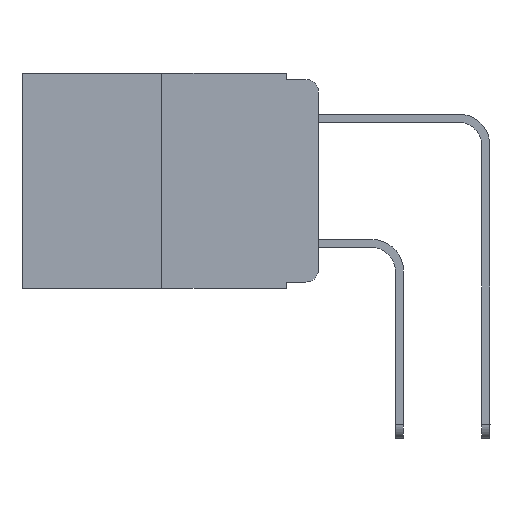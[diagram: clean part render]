
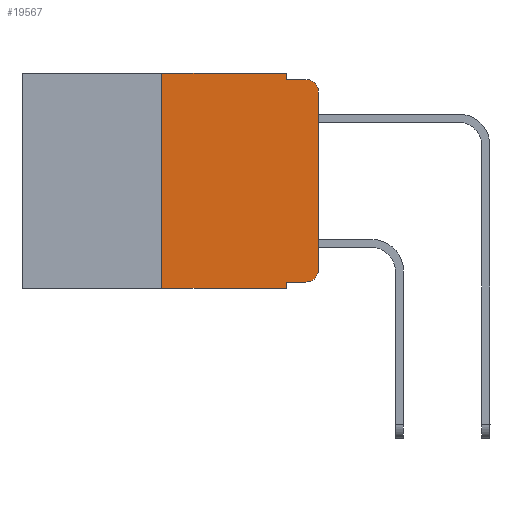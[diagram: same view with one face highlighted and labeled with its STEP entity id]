
A CAD part, left-side view. The second image highlights one B-rep face of the part: STEP entity #19567.
In plain terms, the highlighted planar face has unit normal (-1, 0, 0).
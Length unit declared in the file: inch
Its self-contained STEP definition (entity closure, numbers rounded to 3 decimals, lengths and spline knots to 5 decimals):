
#347 = LINE ( 'NONE', #2165, #15451 ) ;
#647 = EDGE_CURVE ( 'NONE', #5929, #17059, #347, .T. ) ;
#1443 = DIRECTION ( 'NONE',  ( 0., 0., 1. ) ) ;
#1821 = CIRCLE ( 'NONE', #17043, 0.02 ) ;
#1905 = FACE_OUTER_BOUND ( 'NONE', #14694, .T. ) ;
#2043 = DIRECTION ( 'NONE',  ( 0., 0., -1. ) ) ;
#2165 = CARTESIAN_POINT ( 'NONE',  ( 0., 0.051, 0. ) ) ;
#2615 = ORIENTED_EDGE ( 'NONE', *, *, #5912, .T. ) ;
#2757 = CARTESIAN_POINT ( 'NONE',  ( 0., 0.051, 0. ) ) ;
#2917 = CARTESIAN_POINT ( 'NONE',  ( 0., 0., -0.03 ) ) ;
#3136 = ORIENTED_EDGE ( 'NONE', *, *, #7315, .T. ) ;
#3360 = VERTEX_POINT ( 'NONE', #24099 ) ;
#3973 = ORIENTED_EDGE ( 'NONE', *, *, #6894, .T. ) ;
#4538 = CARTESIAN_POINT ( 'NONE',  ( 0., 0.051, -0.333 ) ) ;
#4688 = CARTESIAN_POINT ( 'NONE',  ( 0., 0.473, -0.343 ) ) ;
#4918 = VECTOR ( 'NONE', #14559, 39.37008 ) ;
#5107 = EDGE_CURVE ( 'NONE', #9717, #5424, #20482, .T. ) ;
#5138 = CARTESIAN_POINT ( 'NONE',  ( 0., 0., 0. ) ) ;
#5213 = AXIS2_PLACEMENT_3D ( 'NONE', #23398, #9778, #2043 ) ;
#5356 = CARTESIAN_POINT ( 'NONE',  ( 0., 0.25, -0.343 ) ) ;
#5424 = VERTEX_POINT ( 'NONE', #24143 ) ;
#5912 = EDGE_CURVE ( 'NONE', #24717, #5424, #22689, .T. ) ;
#5929 = VERTEX_POINT ( 'NONE', #2757 ) ;
#6448 = LINE ( 'NONE', #10187, #4918 ) ;
#6863 = CIRCLE ( 'NONE', #5213, 0.02 ) ;
#6894 = EDGE_CURVE ( 'NONE', #9717, #19620, #21118, .T. ) ;
#7283 = VECTOR ( 'NONE', #10864, 39.37008 ) ;
#7315 = EDGE_CURVE ( 'NONE', #17961, #11494, #22758, .T. ) ;
#7467 = PLANE ( 'NONE',  #17533 ) ;
#9049 = ORIENTED_EDGE ( 'NONE', *, *, #19581, .T. ) ;
#9088 = DIRECTION ( 'NONE',  ( -1., 0., 0. ) ) ;
#9091 = LINE ( 'NONE', #14881, #11014 ) ;
#9717 = VERTEX_POINT ( 'NONE', #4538 ) ;
#9778 = DIRECTION ( 'NONE',  ( -1., 0., 0. ) ) ;
#10088 = ORIENTED_EDGE ( 'NONE', *, *, #17295, .T. ) ;
#10187 = CARTESIAN_POINT ( 'NONE',  ( 0., 0.473, 0. ) ) ;
#10258 = CARTESIAN_POINT ( 'NONE',  ( 0., 0.051, -0.01 ) ) ;
#10679 = CARTESIAN_POINT ( 'NONE',  ( 0., 0., -0.313 ) ) ;
#10864 = DIRECTION ( 'NONE',  ( 0., -1., 0. ) ) ;
#10973 = VECTOR ( 'NONE', #23952, 39.37008 ) ;
#11014 = VECTOR ( 'NONE', #16928, 39.37008 ) ;
#11187 = ORIENTED_EDGE ( 'NONE', *, *, #23544, .F. ) ;
#11219 = CARTESIAN_POINT ( 'NONE',  ( 0., 0.051, -0.333 ) ) ;
#11494 = VERTEX_POINT ( 'NONE', #2917 ) ;
#12924 = CARTESIAN_POINT ( 'NONE',  ( 0., 0.25, 0. ) ) ;
#13593 = ORIENTED_EDGE ( 'NONE', *, *, #647, .F. ) ;
#13614 = DIRECTION ( 'NONE',  ( 1., 0., 0. ) ) ;
#14559 = DIRECTION ( 'NONE',  ( 0., -1., 0. ) ) ;
#14580 = EDGE_CURVE ( 'NONE', #24717, #25132, #24877, .T. ) ;
#14694 = EDGE_LOOP ( 'NONE', ( #3136, #9049, #15082, #13593, #11187, #22456, #2615, #15706, #3973, #10088 ) ) ;
#14753 = DIRECTION ( 'NONE',  ( 0., 0., -1. ) ) ;
#14881 = CARTESIAN_POINT ( 'NONE',  ( 0., 0.051, -0.01 ) ) ;
#15082 = ORIENTED_EDGE ( 'NONE', *, *, #21724, .F. ) ;
#15451 = VECTOR ( 'NONE', #23788, 39.37008 ) ;
#15706 = ORIENTED_EDGE ( 'NONE', *, *, #5107, .F. ) ;
#16392 = VECTOR ( 'NONE', #16604, 39.37008 ) ;
#16604 = DIRECTION ( 'NONE',  ( 0., 0., 1. ) ) ;
#16928 = DIRECTION ( 'NONE',  ( 0., -1., 0. ) ) ;
#17043 = AXIS2_PLACEMENT_3D ( 'NONE', #24516, #9088, #14753 ) ;
#17059 = VERTEX_POINT ( 'NONE', #10258 ) ;
#17295 = EDGE_CURVE ( 'NONE', #19620, #17961, #1821, .T. ) ;
#17533 = AXIS2_PLACEMENT_3D ( 'NONE', #19531, #13614, #23152 ) ;
#17961 = VERTEX_POINT ( 'NONE', #10679 ) ;
#18221 = VECTOR ( 'NONE', #1443, 39.37008 ) ;
#19058 = DIRECTION ( 'NONE',  ( 0., -1., 0. ) ) ;
#19531 = CARTESIAN_POINT ( 'NONE',  ( 0., 0.473, 0. ) ) ;
#19567 = ADVANCED_FACE ( 'NONE', ( #1905 ), #7467, .F. ) ;
#19581 = EDGE_CURVE ( 'NONE', #11494, #3360, #6863, .T. ) ;
#19620 = VERTEX_POINT ( 'NONE', #23663 ) ;
#20482 = LINE ( 'NONE', #22410, #10973 ) ;
#21020 = CARTESIAN_POINT ( 'NONE',  ( 0., 0.25, 0. ) ) ;
#21118 = LINE ( 'NONE', #11219, #21697 ) ;
#21697 = VECTOR ( 'NONE', #19058, 39.37008 ) ;
#21724 = EDGE_CURVE ( 'NONE', #17059, #3360, #9091, .T. ) ;
#22410 = CARTESIAN_POINT ( 'NONE',  ( 0., 0.051, 0. ) ) ;
#22456 = ORIENTED_EDGE ( 'NONE', *, *, #14580, .F. ) ;
#22689 = LINE ( 'NONE', #4688, #7283 ) ;
#22758 = LINE ( 'NONE', #5138, #16392 ) ;
#23152 = DIRECTION ( 'NONE',  ( 0., 0., -1. ) ) ;
#23398 = CARTESIAN_POINT ( 'NONE',  ( 0., 0.02, -0.03 ) ) ;
#23544 = EDGE_CURVE ( 'NONE', #25132, #5929, #6448, .T. ) ;
#23663 = CARTESIAN_POINT ( 'NONE',  ( 0., 0.02, -0.333 ) ) ;
#23788 = DIRECTION ( 'NONE',  ( 0., 0., -1. ) ) ;
#23952 = DIRECTION ( 'NONE',  ( 0., 0., -1. ) ) ;
#24099 = CARTESIAN_POINT ( 'NONE',  ( 0., 0.02, -0.01 ) ) ;
#24143 = CARTESIAN_POINT ( 'NONE',  ( 0., 0.051, -0.343 ) ) ;
#24516 = CARTESIAN_POINT ( 'NONE',  ( 0., 0.02, -0.313 ) ) ;
#24717 = VERTEX_POINT ( 'NONE', #5356 ) ;
#24877 = LINE ( 'NONE', #21020, #18221 ) ;
#25132 = VERTEX_POINT ( 'NONE', #12924 ) ;
